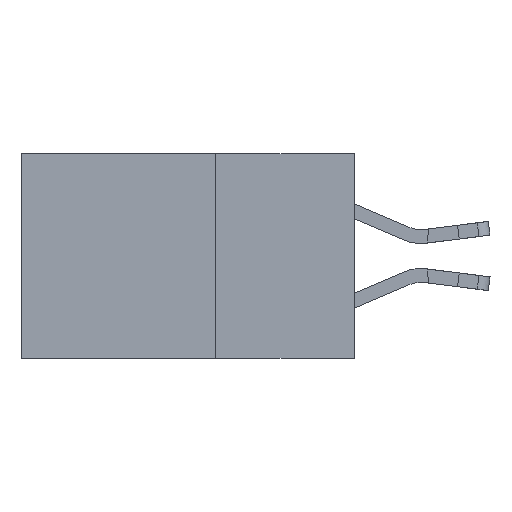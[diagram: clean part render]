
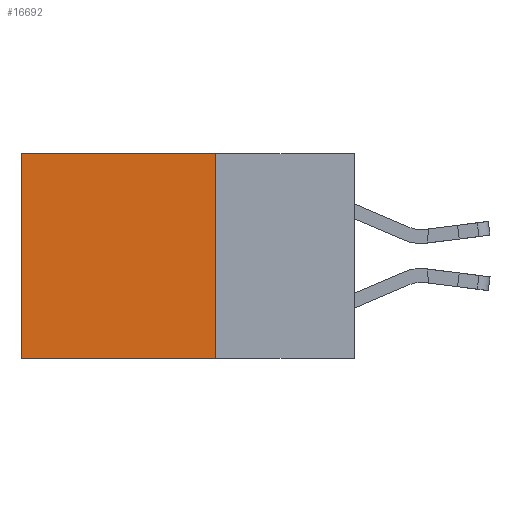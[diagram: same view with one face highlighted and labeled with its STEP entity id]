
A CAD part, left-side view. The second image highlights one B-rep face of the part: STEP entity #16692.
In plain terms, the highlighted planar face has unit normal (-1, 0, 0).
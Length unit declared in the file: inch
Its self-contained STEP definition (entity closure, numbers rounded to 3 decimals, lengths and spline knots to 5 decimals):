
#200 = LINE ( 'NONE', #405, #7710 ) ;
#405 = CARTESIAN_POINT ( 'NONE',  ( 0.2615, 0.25, -0.37 ) ) ;
#905 = AXIS2_PLACEMENT_3D ( 'NONE', #15183, #6687, #16584 ) ;
#1000 = EDGE_CURVE ( 'NONE', #15036, #18246, #17553, .T. ) ;
#1052 = FACE_OUTER_BOUND ( 'NONE', #9151, .T. ) ;
#1151 = ORIENTED_EDGE ( 'NONE', *, *, #1000, .T. ) ;
#2130 = PLANE ( 'NONE',  #905 ) ;
#2303 = LINE ( 'NONE', #10411, #9290 ) ;
#3055 = DIRECTION ( 'NONE',  ( 0., 0., -1. ) ) ;
#3463 = EDGE_CURVE ( 'NONE', #15036, #4954, #6597, .T. ) ;
#4854 = CARTESIAN_POINT ( 'NONE',  ( 0.2615, 0.25, 0. ) ) ;
#4880 = DIRECTION ( 'NONE',  ( 0., 1., 0. ) ) ;
#4954 = VERTEX_POINT ( 'NONE', #7146 ) ;
#6209 = VECTOR ( 'NONE', #4880, 39.37008 ) ;
#6597 = LINE ( 'NONE', #13700, #13729 ) ;
#6687 = DIRECTION ( 'NONE',  ( 1., 0., 0. ) ) ;
#7146 = CARTESIAN_POINT ( 'NONE',  ( 0.2615, 0.25, -0.37 ) ) ;
#7395 = ORIENTED_EDGE ( 'NONE', *, *, #3463, .F. ) ;
#7710 = VECTOR ( 'NONE', #12175, 39.37008 ) ;
#9151 = EDGE_LOOP ( 'NONE', ( #12765, #18180, #7395, #1151 ) ) ;
#9290 = VECTOR ( 'NONE', #3055, 39.37008 ) ;
#10411 = CARTESIAN_POINT ( 'NONE',  ( 0.2615, 0.6, -0.37 ) ) ;
#11677 = VERTEX_POINT ( 'NONE', #18789 ) ;
#12175 = DIRECTION ( 'NONE',  ( 0., 1., 0. ) ) ;
#12765 = ORIENTED_EDGE ( 'NONE', *, *, #14148, .T. ) ;
#13088 = EDGE_CURVE ( 'NONE', #4954, #11677, #200, .T. ) ;
#13139 = DIRECTION ( 'NONE',  ( 0., 0., -1. ) ) ;
#13700 = CARTESIAN_POINT ( 'NONE',  ( 0.2615, 0.25, -0.37 ) ) ;
#13729 = VECTOR ( 'NONE', #13139, 39.37008 ) ;
#14148 = EDGE_CURVE ( 'NONE', #18246, #11677, #2303, .T. ) ;
#14207 = CARTESIAN_POINT ( 'NONE',  ( 0.2615, 0.6, 0. ) ) ;
#15036 = VERTEX_POINT ( 'NONE', #17744 ) ;
#15183 = CARTESIAN_POINT ( 'NONE',  ( 0.2615, 0.25, -0.37 ) ) ;
#16584 = DIRECTION ( 'NONE',  ( 0., 0., -1. ) ) ;
#16692 = ADVANCED_FACE ( 'NONE', ( #1052 ), #2130, .F. ) ;
#17553 = LINE ( 'NONE', #4854, #6209 ) ;
#17744 = CARTESIAN_POINT ( 'NONE',  ( 0.2615, 0.25, 0. ) ) ;
#18180 = ORIENTED_EDGE ( 'NONE', *, *, #13088, .F. ) ;
#18246 = VERTEX_POINT ( 'NONE', #14207 ) ;
#18789 = CARTESIAN_POINT ( 'NONE',  ( 0.2615, 0.6, -0.37 ) ) ;
